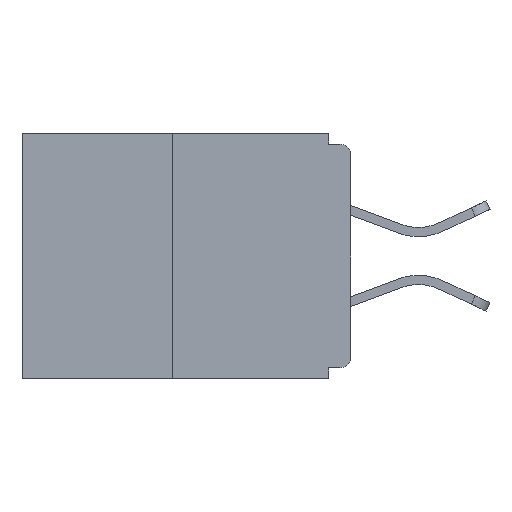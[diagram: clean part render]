
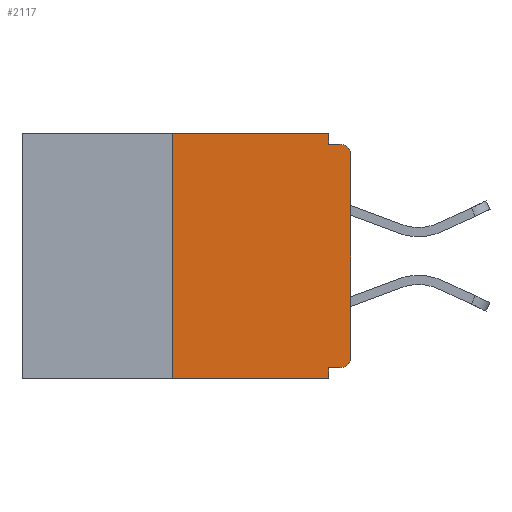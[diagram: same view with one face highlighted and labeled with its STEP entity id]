
A CAD part, left-side view. The second image highlights one B-rep face of the part: STEP entity #2117.
In plain terms, the highlighted planar face has unit normal (-1, 0, 0).
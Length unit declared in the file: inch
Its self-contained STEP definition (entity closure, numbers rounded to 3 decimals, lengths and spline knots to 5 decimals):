
#444 = VERTEX_POINT ( 'NONE', #15066 ) ;
#466 = EDGE_CURVE ( 'NONE', #14055, #17116, #19990, .T. ) ;
#635 = DIRECTION ( 'NONE',  ( 0., 0., -1. ) ) ;
#862 = VECTOR ( 'NONE', #10398, 39.37008 ) ;
#1170 = CARTESIAN_POINT ( 'NONE',  ( 0., 0.031, -0.015 ) ) ;
#1349 = DIRECTION ( 'NONE',  ( 0., 0., -1. ) ) ;
#1443 = ORIENTED_EDGE ( 'NONE', *, *, #5201, .T. ) ;
#1457 = ORIENTED_EDGE ( 'NONE', *, *, #2288, .F. ) ;
#1703 = AXIS2_PLACEMENT_3D ( 'NONE', #4772, #16190, #6433 ) ;
#1822 = EDGE_CURVE ( 'NONE', #17116, #2071, #13597, .T. ) ;
#1861 = CIRCLE ( 'NONE', #19809, 0.015 ) ;
#2043 = CARTESIAN_POINT ( 'NONE',  ( 0., 0., -0.03 ) ) ;
#2071 = VERTEX_POINT ( 'NONE', #14903 ) ;
#2117 = ADVANCED_FACE ( 'NONE', ( #9776 ), #20729, .F. ) ;
#2128 = DIRECTION ( 'NONE',  ( 0., 0., -1. ) ) ;
#2221 = EDGE_LOOP ( 'NONE', ( #12740, #15380, #1443, #13249, #9812, #13688, #16812, #5370, #10701, #1457 ) ) ;
#2288 = EDGE_CURVE ( 'NONE', #2071, #3078, #19718, .T. ) ;
#3078 = VERTEX_POINT ( 'NONE', #1170 ) ;
#3504 = LINE ( 'NONE', #15220, #20326 ) ;
#4772 = CARTESIAN_POINT ( 'NONE',  ( 0., 0.015, -0.03 ) ) ;
#4846 = CARTESIAN_POINT ( 'NONE',  ( 0., 0., 0. ) ) ;
#5201 = EDGE_CURVE ( 'NONE', #14055, #16220, #14191, .T. ) ;
#5206 = CARTESIAN_POINT ( 'NONE',  ( 0., 0.25, 0. ) ) ;
#5370 = ORIENTED_EDGE ( 'NONE', *, *, #18153, .T. ) ;
#5379 = DIRECTION ( 'NONE',  ( 0., -1., 0. ) ) ;
#5403 = VECTOR ( 'NONE', #11525, 39.37008 ) ;
#5511 = CARTESIAN_POINT ( 'NONE',  ( 0., 0.015, -0.313 ) ) ;
#5681 = VERTEX_POINT ( 'NONE', #7591 ) ;
#5834 = CARTESIAN_POINT ( 'NONE',  ( 0., 0.015, -0.328 ) ) ;
#6039 = EDGE_CURVE ( 'NONE', #444, #14292, #7784, .T. ) ;
#6365 = EDGE_CURVE ( 'NONE', #12710, #13281, #8555, .T. ) ;
#6433 = DIRECTION ( 'NONE',  ( 0., 0., -1. ) ) ;
#7457 = CIRCLE ( 'NONE', #1703, 0.015 ) ;
#7591 = CARTESIAN_POINT ( 'NONE',  ( 0., 0.015, -0.015 ) ) ;
#7784 = LINE ( 'NONE', #4846, #18761 ) ;
#8235 = CARTESIAN_POINT ( 'NONE',  ( 0., 0.46, 0. ) ) ;
#8520 = VECTOR ( 'NONE', #11211, 39.37008 ) ;
#8555 = LINE ( 'NONE', #11834, #862 ) ;
#9370 = EDGE_CURVE ( 'NONE', #13281, #16220, #3504, .T. ) ;
#9488 = AXIS2_PLACEMENT_3D ( 'NONE', #11192, #12844, #1349 ) ;
#9776 = FACE_OUTER_BOUND ( 'NONE', #2221, .T. ) ;
#9812 = ORIENTED_EDGE ( 'NONE', *, *, #6365, .F. ) ;
#9830 = CARTESIAN_POINT ( 'NONE',  ( 0., 0.25, 0. ) ) ;
#10208 = CARTESIAN_POINT ( 'NONE',  ( 0., 0.46, -0.343 ) ) ;
#10251 = VECTOR ( 'NONE', #18332, 39.37008 ) ;
#10398 = DIRECTION ( 'NONE',  ( 0., 1., 0. ) ) ;
#10533 = DIRECTION ( 'NONE',  ( -1., 0., 0. ) ) ;
#10701 = ORIENTED_EDGE ( 'NONE', *, *, #12925, .F. ) ;
#11192 = CARTESIAN_POINT ( 'NONE',  ( 0., 0.46, 0. ) ) ;
#11211 = DIRECTION ( 'NONE',  ( 0., -1., 0. ) ) ;
#11472 = DIRECTION ( 'NONE',  ( 0., 0., 1. ) ) ;
#11525 = DIRECTION ( 'NONE',  ( 0., -1., 0. ) ) ;
#11834 = CARTESIAN_POINT ( 'NONE',  ( 0., 0., -0.328 ) ) ;
#12710 = VERTEX_POINT ( 'NONE', #5834 ) ;
#12740 = ORIENTED_EDGE ( 'NONE', *, *, #1822, .F. ) ;
#12844 = DIRECTION ( 'NONE',  ( 1., 0., 0. ) ) ;
#12925 = EDGE_CURVE ( 'NONE', #3078, #5681, #18409, .T. ) ;
#13095 = CARTESIAN_POINT ( 'NONE',  ( 0., 0.031, -0.343 ) ) ;
#13249 = ORIENTED_EDGE ( 'NONE', *, *, #9370, .F. ) ;
#13269 = CARTESIAN_POINT ( 'NONE',  ( 0., 0.031, 0. ) ) ;
#13281 = VERTEX_POINT ( 'NONE', #15331 ) ;
#13597 = LINE ( 'NONE', #8235, #8520 ) ;
#13681 = EDGE_CURVE ( 'NONE', #12710, #444, #1861, .T. ) ;
#13688 = ORIENTED_EDGE ( 'NONE', *, *, #13681, .T. ) ;
#14055 = VERTEX_POINT ( 'NONE', #17980 ) ;
#14191 = LINE ( 'NONE', #10208, #18076 ) ;
#14292 = VERTEX_POINT ( 'NONE', #2043 ) ;
#14854 = CARTESIAN_POINT ( 'NONE',  ( 0., 0., -0.015 ) ) ;
#14903 = CARTESIAN_POINT ( 'NONE',  ( 0., 0.031, 0. ) ) ;
#15066 = CARTESIAN_POINT ( 'NONE',  ( 0., 0., -0.313 ) ) ;
#15220 = CARTESIAN_POINT ( 'NONE',  ( 0., 0.031, -0.343 ) ) ;
#15331 = CARTESIAN_POINT ( 'NONE',  ( 0., 0.031, -0.328 ) ) ;
#15380 = ORIENTED_EDGE ( 'NONE', *, *, #466, .F. ) ;
#16190 = DIRECTION ( 'NONE',  ( -1., 0., 0. ) ) ;
#16220 = VERTEX_POINT ( 'NONE', #13095 ) ;
#16812 = ORIENTED_EDGE ( 'NONE', *, *, #6039, .T. ) ;
#17116 = VERTEX_POINT ( 'NONE', #9830 ) ;
#17452 = VECTOR ( 'NONE', #18388, 39.37008 ) ;
#17980 = CARTESIAN_POINT ( 'NONE',  ( 0., 0.25, -0.343 ) ) ;
#18076 = VECTOR ( 'NONE', #5379, 39.37008 ) ;
#18153 = EDGE_CURVE ( 'NONE', #14292, #5681, #7457, .T. ) ;
#18332 = DIRECTION ( 'NONE',  ( 0., 0., -1. ) ) ;
#18388 = DIRECTION ( 'NONE',  ( 0., 0., 1. ) ) ;
#18409 = LINE ( 'NONE', #14854, #5403 ) ;
#18761 = VECTOR ( 'NONE', #11472, 39.37008 ) ;
#19718 = LINE ( 'NONE', #13269, #10251 ) ;
#19809 = AXIS2_PLACEMENT_3D ( 'NONE', #5511, #10533, #635 ) ;
#19990 = LINE ( 'NONE', #5206, #17452 ) ;
#20326 = VECTOR ( 'NONE', #2128, 39.37008 ) ;
#20729 = PLANE ( 'NONE',  #9488 ) ;
